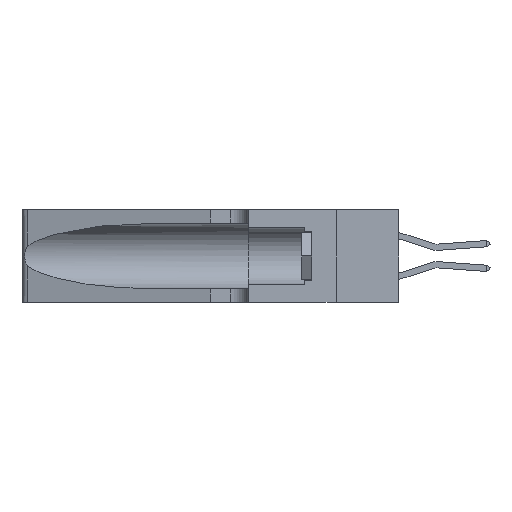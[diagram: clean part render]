
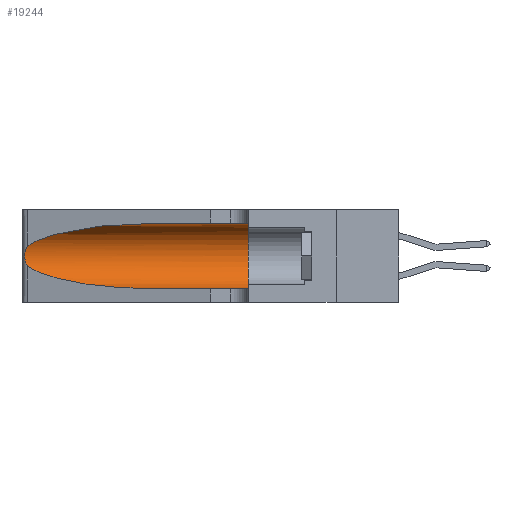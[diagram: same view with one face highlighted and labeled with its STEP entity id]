
A CAD part, left-side view. The second image highlights one B-rep face of the part: STEP entity #19244.
In plain terms, the highlighted cylindrical face has radius 3.308 mm (diameter 6.617 mm), a partial arc.
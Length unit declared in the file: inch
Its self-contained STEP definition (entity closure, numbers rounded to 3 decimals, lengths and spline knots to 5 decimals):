
#51 = EDGE_LOOP ( 'NONE', ( #14106, #18449, #8984, #13438, #10913, #7819 ) ) ;
#711 = CARTESIAN_POINT ( 'NONE',  ( 0.1305, 0.72297, 0.05475 ) ) ;
#986 = B_SPLINE_CURVE_WITH_KNOTS ( 'NONE', 3,
 ( #5932, #7421, #17785, #8937, #19246, #10484, #1210, #11982, #2839, #13454, #4461, #14919, #5994, #16376 ),
 .UNSPECIFIED., .F., .F.,
 ( 4, 2, 2, 2, 2, 2, 4 ),
 ( 0., 0.00027, 0.00053, 0.00107, 0.0016, 0.00187, 0.00214 ),
 .UNSPECIFIED. ) ;
#1143 =( BOUNDED_CURVE ( )  B_SPLINE_CURVE ( 3, ( #18992, #16058, #4164, #14654 ),
 .UNSPECIFIED., .F., .F. ) 
 B_SPLINE_CURVE_WITH_KNOTS ( ( 4, 4 ),
 ( 1.5708, 2.84003 ),
 .UNSPECIFIED. ) 
 CURVE ( )  GEOMETRIC_REPRESENTATION_ITEM ( )  RATIONAL_B_SPLINE_CURVE ( ( 1., 0.87, 0.87, 1. ) ) 
 REPRESENTATION_ITEM ( '' )  );
#1177 = VERTEX_POINT ( 'NONE', #6900 ) ;
#1210 = CARTESIAN_POINT ( 'NONE',  ( 0.26075, 1.23896, 0.19203 ) ) ;
#1464 = VERTEX_POINT ( 'NONE', #10302 ) ;
#1489 = VECTOR ( 'NONE', #4939, 39.37008 ) ;
#2171 = AXIS2_PLACEMENT_3D ( 'NONE', #16336, #7449, #8958 ) ;
#2497 = LINE ( 'NONE', #18177, #1489 ) ;
#2831 =( BOUNDED_CURVE ( )  B_SPLINE_CURVE ( 3, ( #10050, #9988, #8512, #711 ),
 .UNSPECIFIED., .F., .T. ) 
 B_SPLINE_CURVE_WITH_KNOTS ( ( 4, 4 ),
 ( 3.44316, 4.71239 ),
 .UNSPECIFIED. ) 
 CURVE ( )  GEOMETRIC_REPRESENTATION_ITEM ( )  RATIONAL_B_SPLINE_CURVE ( ( 1., 0.87, 0.87, 1. ) ) 
 REPRESENTATION_ITEM ( '' )  );
#2839 = CARTESIAN_POINT ( 'NONE',  ( 0.26017, 1.23833, 0.17102 ) ) ;
#3828 = CARTESIAN_POINT ( 'NONE',  ( 0.1305, 1.61858, 0.05475 ) ) ;
#4164 = CARTESIAN_POINT ( 'NONE',  ( 0.2373, 1.15595, 0.28018 ) ) ;
#4440 = CIRCLE ( 'NONE', #15048, 0.13025 ) ;
#4461 = CARTESIAN_POINT ( 'NONE',  ( 0.25789, 1.23486, 0.15765 ) ) ;
#4939 = DIRECTION ( 'NONE',  ( 0., -1., 0. ) ) ;
#5858 = EDGE_CURVE ( 'NONE', #7314, #13819, #2831, .T. ) ;
#5932 = CARTESIAN_POINT ( 'NONE',  ( 0.25487, 1.22718, 0.22369 ) ) ;
#5994 = CARTESIAN_POINT ( 'NONE',  ( 0.25555, 1.22993, 0.14849 ) ) ;
#6161 = LINE ( 'NONE', #3828, #17982 ) ;
#6674 = EDGE_CURVE ( 'NONE', #11638, #1464, #2497, .T. ) ;
#6900 = CARTESIAN_POINT ( 'NONE',  ( 0.25487, 1.22718, 0.22369 ) ) ;
#7314 = VERTEX_POINT ( 'NONE', #19541 ) ;
#7421 = CARTESIAN_POINT ( 'NONE',  ( 0.25555, 1.22994, 0.2215 ) ) ;
#7449 = DIRECTION ( 'NONE',  ( 0., -1., 0. ) ) ;
#7819 = ORIENTED_EDGE ( 'NONE', *, *, #6674, .F. ) ;
#8494 = FACE_OUTER_BOUND ( 'NONE', #51, .T. ) ;
#8512 = CARTESIAN_POINT ( 'NONE',  ( 0.18966, 0.96281, 0.05475 ) ) ;
#8754 = DIRECTION ( 'NONE',  ( 0., 1., 0. ) ) ;
#8937 = CARTESIAN_POINT ( 'NONE',  ( 0.25787, 1.23484, 0.2124 ) ) ;
#8958 = DIRECTION ( 'NONE',  ( 0., 0., -1. ) ) ;
#8984 = ORIENTED_EDGE ( 'NONE', *, *, #5858, .T. ) ;
#9988 = CARTESIAN_POINT ( 'NONE',  ( 0.2373, 1.15595, 0.08982 ) ) ;
#10050 = CARTESIAN_POINT ( 'NONE',  ( 0.25487, 1.22718, 0.14631 ) ) ;
#10302 = CARTESIAN_POINT ( 'NONE',  ( 0.1305, 0.35, 0.31525 ) ) ;
#10484 = CARTESIAN_POINT ( 'NONE',  ( 0.26018, 1.23835, 0.19895 ) ) ;
#10913 = ORIENTED_EDGE ( 'NONE', *, *, #14556, .F. ) ;
#11127 = VERTEX_POINT ( 'NONE', #18211 ) ;
#11573 = CYLINDRICAL_SURFACE ( 'NONE', #2171, 0.13025 ) ;
#11638 = VERTEX_POINT ( 'NONE', #17814 ) ;
#11982 = CARTESIAN_POINT ( 'NONE',  ( 0.26075, 1.23896, 0.178 ) ) ;
#13438 = ORIENTED_EDGE ( 'NONE', *, *, #13793, .T. ) ;
#13454 = CARTESIAN_POINT ( 'NONE',  ( 0.25856, 1.23593, 0.16098 ) ) ;
#13793 = EDGE_CURVE ( 'NONE', #13819, #11127, #6161, .T. ) ;
#13819 = VERTEX_POINT ( 'NONE', #15816 ) ;
#13937 = EDGE_CURVE ( 'NONE', #11638, #1177, #1143, .T. ) ;
#14106 = ORIENTED_EDGE ( 'NONE', *, *, #13937, .T. ) ;
#14340 = DIRECTION ( 'NONE',  ( 0., -1., 0. ) ) ;
#14556 = EDGE_CURVE ( 'NONE', #1464, #11127, #4440, .T. ) ;
#14654 = CARTESIAN_POINT ( 'NONE',  ( 0.25487, 1.22718, 0.22369 ) ) ;
#14919 = CARTESIAN_POINT ( 'NONE',  ( 0.25639, 1.23186, 0.15144 ) ) ;
#15048 = AXIS2_PLACEMENT_3D ( 'NONE', #17598, #8754, #19070 ) ;
#15816 = CARTESIAN_POINT ( 'NONE',  ( 0.1305, 0.72297, 0.05475 ) ) ;
#16058 = CARTESIAN_POINT ( 'NONE',  ( 0.18966, 0.96281, 0.31525 ) ) ;
#16336 = CARTESIAN_POINT ( 'NONE',  ( 0.1305, 1.61858, 0.185 ) ) ;
#16376 = CARTESIAN_POINT ( 'NONE',  ( 0.25487, 1.22718, 0.14631 ) ) ;
#16587 = EDGE_CURVE ( 'NONE', #1177, #7314, #986, .T. ) ;
#17598 = CARTESIAN_POINT ( 'NONE',  ( 0.1305, 0.35, 0.185 ) ) ;
#17785 = CARTESIAN_POINT ( 'NONE',  ( 0.25639, 1.23184, 0.21858 ) ) ;
#17814 = CARTESIAN_POINT ( 'NONE',  ( 0.1305, 0.72297, 0.31525 ) ) ;
#17982 = VECTOR ( 'NONE', #14340, 39.37008 ) ;
#18177 = CARTESIAN_POINT ( 'NONE',  ( 0.1305, 1.61858, 0.31525 ) ) ;
#18211 = CARTESIAN_POINT ( 'NONE',  ( 0.1305, 0.35, 0.05475 ) ) ;
#18449 = ORIENTED_EDGE ( 'NONE', *, *, #16587, .T. ) ;
#18992 = CARTESIAN_POINT ( 'NONE',  ( 0.1305, 0.72297, 0.31525 ) ) ;
#19070 = DIRECTION ( 'NONE',  ( 0., 0., 1. ) ) ;
#19244 = ADVANCED_FACE ( 'NONE', ( #8494 ), #11573, .F. ) ;
#19246 = CARTESIAN_POINT ( 'NONE',  ( 0.25854, 1.2359, 0.20912 ) ) ;
#19541 = CARTESIAN_POINT ( 'NONE',  ( 0.25487, 1.22718, 0.14631 ) ) ;
